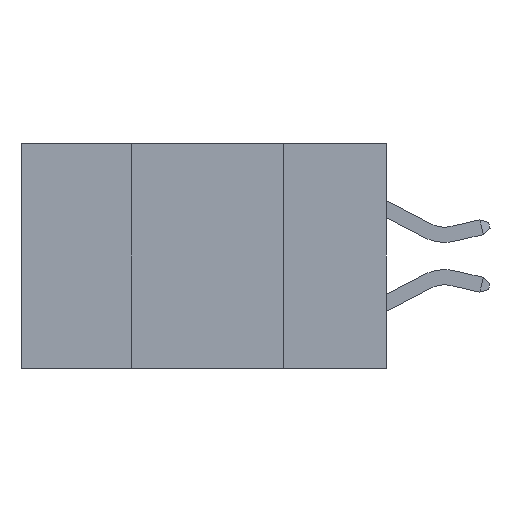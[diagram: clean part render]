
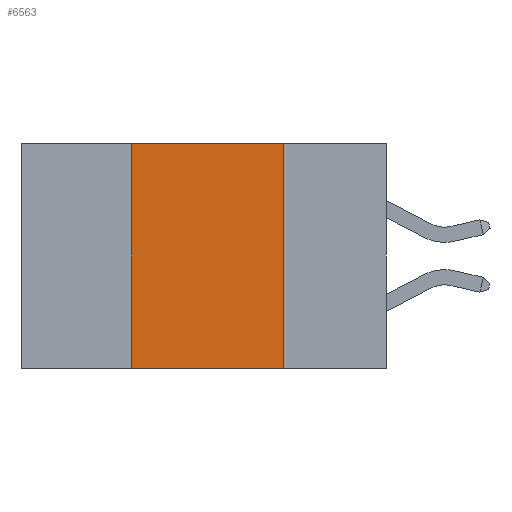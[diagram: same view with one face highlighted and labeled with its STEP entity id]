
A CAD part, left-side view. The second image highlights one B-rep face of the part: STEP entity #6563.
In plain terms, the highlighted planar face has unit normal (-1, 0, 0).
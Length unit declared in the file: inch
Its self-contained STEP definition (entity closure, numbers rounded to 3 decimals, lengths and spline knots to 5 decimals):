
#415 = VERTEX_POINT ( 'NONE', #2861 ) ;
#448 = VECTOR ( 'NONE', #4355, 39.37008 ) ;
#904 = LINE ( 'NONE', #12574, #18518 ) ;
#1039 = DIRECTION ( 'NONE',  ( 1., 0., 0. ) ) ;
#1384 = AXIS2_PLACEMENT_3D ( 'NONE', #24419, #1039, #24295 ) ;
#2748 = EDGE_CURVE ( 'NONE', #12787, #14227, #7109, .T. ) ;
#2861 = CARTESIAN_POINT ( 'NONE',  ( 0., 0.42, -0.37 ) ) ;
#4355 = DIRECTION ( 'NONE',  ( 0., -1., 0. ) ) ;
#5719 = VECTOR ( 'NONE', #14216, 39.37008 ) ;
#6563 = ADVANCED_FACE ( 'NONE', ( #16567 ), #10520, .F. ) ;
#7109 = LINE ( 'NONE', #22508, #9518 ) ;
#7641 = ORIENTED_EDGE ( 'NONE', *, *, #23561, .F. ) ;
#8540 = CARTESIAN_POINT ( 'NONE',  ( 0., 0.17, -0.37 ) ) ;
#9518 = VECTOR ( 'NONE', #24832, 39.37008 ) ;
#10288 = EDGE_CURVE ( 'NONE', #415, #14227, #14122, .T. ) ;
#10517 = DIRECTION ( 'NONE',  ( 0., -1., 0. ) ) ;
#10520 = PLANE ( 'NONE',  #1384 ) ;
#12469 = ORIENTED_EDGE ( 'NONE', *, *, #10288, .T. ) ;
#12574 = CARTESIAN_POINT ( 'NONE',  ( 0., 0.6, 0. ) ) ;
#12787 = VERTEX_POINT ( 'NONE', #14563 ) ;
#14122 = LINE ( 'NONE', #21954, #448 ) ;
#14216 = DIRECTION ( 'NONE',  ( 0., 0., 1. ) ) ;
#14227 = VERTEX_POINT ( 'NONE', #8540 ) ;
#14563 = CARTESIAN_POINT ( 'NONE',  ( 0., 0.17, 0. ) ) ;
#14866 = CARTESIAN_POINT ( 'NONE',  ( 0., 0.42, 0. ) ) ;
#16567 = FACE_OUTER_BOUND ( 'NONE', #18966, .T. ) ;
#16979 = EDGE_CURVE ( 'NONE', #22964, #12787, #904, .T. ) ;
#17946 = ORIENTED_EDGE ( 'NONE', *, *, #2748, .F. ) ;
#18518 = VECTOR ( 'NONE', #10517, 39.37008 ) ;
#18966 = EDGE_LOOP ( 'NONE', ( #17946, #22030, #7641, #12469 ) ) ;
#21954 = CARTESIAN_POINT ( 'NONE',  ( 0., 0.6, -0.37 ) ) ;
#22030 = ORIENTED_EDGE ( 'NONE', *, *, #16979, .F. ) ;
#22046 = CARTESIAN_POINT ( 'NONE',  ( 0., 0.42, -0.37 ) ) ;
#22182 = LINE ( 'NONE', #22046, #5719 ) ;
#22508 = CARTESIAN_POINT ( 'NONE',  ( 0., 0.17, -0.37 ) ) ;
#22964 = VERTEX_POINT ( 'NONE', #14866 ) ;
#23561 = EDGE_CURVE ( 'NONE', #415, #22964, #22182, .T. ) ;
#24295 = DIRECTION ( 'NONE',  ( 0., 0., -1. ) ) ;
#24419 = CARTESIAN_POINT ( 'NONE',  ( 0., 0.6, 0. ) ) ;
#24832 = DIRECTION ( 'NONE',  ( 0., 0., -1. ) ) ;
